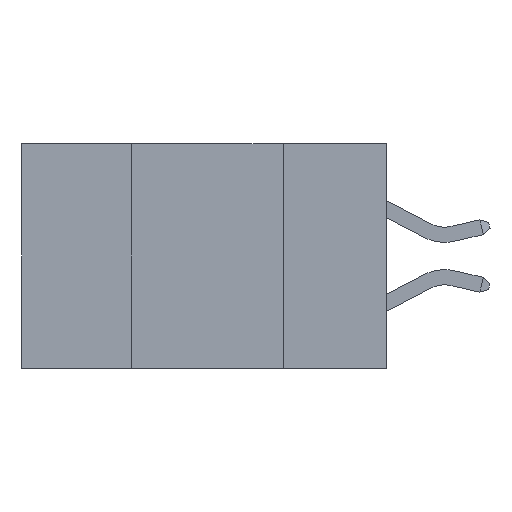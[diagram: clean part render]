
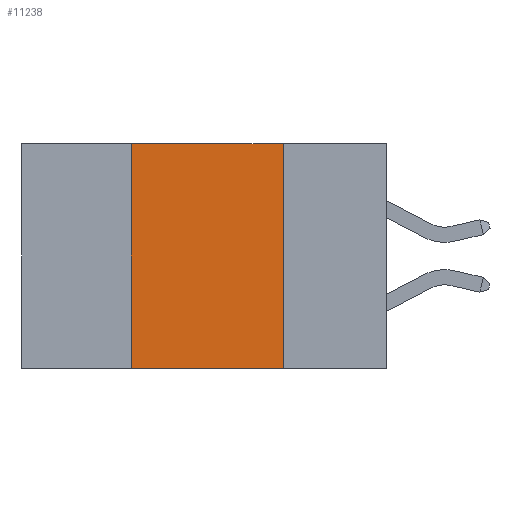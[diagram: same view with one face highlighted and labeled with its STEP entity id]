
A CAD part, left-side view. The second image highlights one B-rep face of the part: STEP entity #11238.
In plain terms, the highlighted planar face has unit normal (-1, 0, 0).
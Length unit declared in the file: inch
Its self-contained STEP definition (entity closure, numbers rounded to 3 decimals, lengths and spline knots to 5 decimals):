
#797 = ORIENTED_EDGE ( 'NONE', *, *, #10707, .T. ) ;
#899 = EDGE_CURVE ( 'NONE', #1180, #3435, #7760, .T. ) ;
#1180 = VERTEX_POINT ( 'NONE', #3686 ) ;
#2850 = CARTESIAN_POINT ( 'NONE',  ( 0., 0.42, -0.37 ) ) ;
#2869 = VECTOR ( 'NONE', #8622, 39.37008 ) ;
#2969 = FACE_OUTER_BOUND ( 'NONE', #4270, .T. ) ;
#2998 = CARTESIAN_POINT ( 'NONE',  ( 0., 0.17, 0. ) ) ;
#3435 = VERTEX_POINT ( 'NONE', #8486 ) ;
#3686 = CARTESIAN_POINT ( 'NONE',  ( 0., 0.17, 0. ) ) ;
#3828 = CARTESIAN_POINT ( 'NONE',  ( 0., 0.6, -0.37 ) ) ;
#4002 = VERTEX_POINT ( 'NONE', #2850 ) ;
#4270 = EDGE_LOOP ( 'NONE', ( #6199, #6028, #10285, #797 ) ) ;
#4403 = EDGE_CURVE ( 'NONE', #5036, #1180, #8331, .T. ) ;
#4572 = DIRECTION ( 'NONE',  ( 1., 0., 0. ) ) ;
#4753 = VECTOR ( 'NONE', #9977, 39.37008 ) ;
#5036 = VERTEX_POINT ( 'NONE', #9021 ) ;
#5464 = LINE ( 'NONE', #11432, #7847 ) ;
#5469 = PLANE ( 'NONE',  #8983 ) ;
#5511 = DIRECTION ( 'NONE',  ( 0., 0., 1. ) ) ;
#6028 = ORIENTED_EDGE ( 'NONE', *, *, #4403, .F. ) ;
#6199 = ORIENTED_EDGE ( 'NONE', *, *, #899, .F. ) ;
#6381 = CARTESIAN_POINT ( 'NONE',  ( 0., 0.6, 0. ) ) ;
#6880 = LINE ( 'NONE', #3828, #4753 ) ;
#7760 = LINE ( 'NONE', #2998, #2869 ) ;
#7847 = VECTOR ( 'NONE', #5511, 39.37008 ) ;
#8331 = LINE ( 'NONE', #6381, #9985 ) ;
#8486 = CARTESIAN_POINT ( 'NONE',  ( 0., 0.17, -0.37 ) ) ;
#8622 = DIRECTION ( 'NONE',  ( 0., 0., -1. ) ) ;
#8983 = AXIS2_PLACEMENT_3D ( 'NONE', #9778, #4572, #10616 ) ;
#9021 = CARTESIAN_POINT ( 'NONE',  ( 0., 0.42, 0. ) ) ;
#9358 = DIRECTION ( 'NONE',  ( 0., -1., 0. ) ) ;
#9778 = CARTESIAN_POINT ( 'NONE',  ( 0., 0.6, 0. ) ) ;
#9977 = DIRECTION ( 'NONE',  ( 0., -1., 0. ) ) ;
#9985 = VECTOR ( 'NONE', #9358, 39.37008 ) ;
#10285 = ORIENTED_EDGE ( 'NONE', *, *, #11243, .F. ) ;
#10616 = DIRECTION ( 'NONE',  ( 0., 0., -1. ) ) ;
#10707 = EDGE_CURVE ( 'NONE', #4002, #3435, #6880, .T. ) ;
#11238 = ADVANCED_FACE ( 'NONE', ( #2969 ), #5469, .F. ) ;
#11243 = EDGE_CURVE ( 'NONE', #4002, #5036, #5464, .T. ) ;
#11432 = CARTESIAN_POINT ( 'NONE',  ( 0., 0.42, 0. ) ) ;
